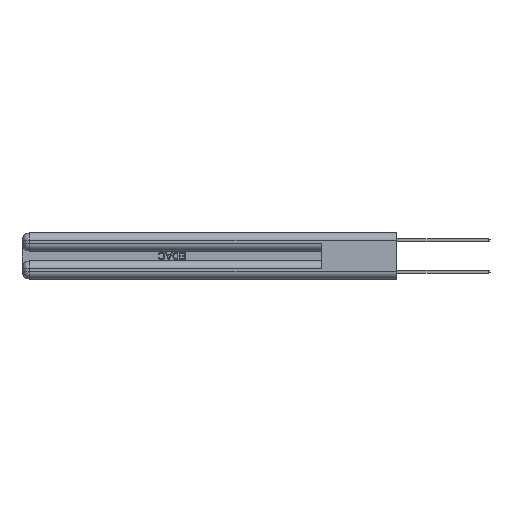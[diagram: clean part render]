
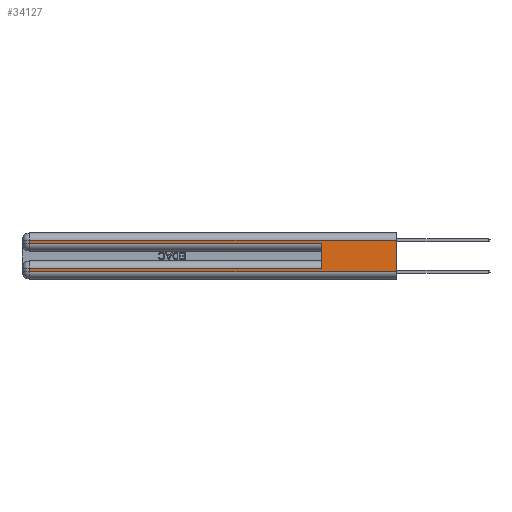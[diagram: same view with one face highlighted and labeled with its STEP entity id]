
A CAD part, left-side view. The second image highlights one B-rep face of the part: STEP entity #34127.
In plain terms, the highlighted planar face has unit normal (-1, 0, 0).
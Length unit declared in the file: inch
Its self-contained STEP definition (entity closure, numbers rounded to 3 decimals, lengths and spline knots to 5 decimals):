
#540 = EDGE_CURVE ( 'NONE', #30576, #14125, #21364, .T. ) ;
#1608 = ORIENTED_EDGE ( 'NONE', *, *, #540, .F. ) ;
#1637 = DIRECTION ( 'NONE',  ( 0., 1., 0. ) ) ;
#1797 = DIRECTION ( 'NONE',  ( 1., 0., 0. ) ) ;
#2330 = CARTESIAN_POINT ( 'NONE',  ( 0., 2.94, 0.31 ) ) ;
#2405 = CARTESIAN_POINT ( 'NONE',  ( 0., 2.94, 0.085 ) ) ;
#2927 = EDGE_LOOP ( 'NONE', ( #27603, #15853, #14263, #14037, #1608, #10735, #12946, #26251 ) ) ;
#3927 = PLANE ( 'NONE',  #29278 ) ;
#5825 = EDGE_CURVE ( 'NONE', #24132, #31583, #33546, .T. ) ;
#5910 = DIRECTION ( 'NONE',  ( 0., 0., -1. ) ) ;
#6086 = CARTESIAN_POINT ( 'NONE',  ( 0., 0., 0.085 ) ) ;
#7013 = DIRECTION ( 'NONE',  ( 0., 0., -1. ) ) ;
#7565 = VECTOR ( 'NONE', #11944, 39.37008 ) ;
#7853 = VECTOR ( 'NONE', #16597, 39.37008 ) ;
#8237 = EDGE_CURVE ( 'NONE', #31583, #25192, #31632, .T. ) ;
#10208 = CARTESIAN_POINT ( 'NONE',  ( 0., 0., 0.31 ) ) ;
#10735 = ORIENTED_EDGE ( 'NONE', *, *, #13315, .T. ) ;
#11313 = VERTEX_POINT ( 'NONE', #2330 ) ;
#11636 = CARTESIAN_POINT ( 'NONE',  ( 0., 0., 0.37 ) ) ;
#11944 = DIRECTION ( 'NONE',  ( 0., 0., -1. ) ) ;
#12946 = ORIENTED_EDGE ( 'NONE', *, *, #5825, .T. ) ;
#13315 = EDGE_CURVE ( 'NONE', #30576, #24132, #30402, .T. ) ;
#13372 = EDGE_CURVE ( 'NONE', #11313, #16018, #21155, .T. ) ;
#13816 = FACE_OUTER_BOUND ( 'NONE', #2927, .T. ) ;
#13921 = DIRECTION ( 'NONE',  ( 0., -1., 0. ) ) ;
#14037 = ORIENTED_EDGE ( 'NONE', *, *, #24887, .T. ) ;
#14125 = VERTEX_POINT ( 'NONE', #23801 ) ;
#14263 = ORIENTED_EDGE ( 'NONE', *, *, #13372, .T. ) ;
#14630 = CARTESIAN_POINT ( 'NONE',  ( 0., 0., 0.285 ) ) ;
#15293 = EDGE_CURVE ( 'NONE', #24166, #11313, #15877, .T. ) ;
#15853 = ORIENTED_EDGE ( 'NONE', *, *, #15293, .T. ) ;
#15877 = LINE ( 'NONE', #10208, #29428 ) ;
#16018 = VERTEX_POINT ( 'NONE', #25874 ) ;
#16597 = DIRECTION ( 'NONE',  ( 0., 0., -1. ) ) ;
#16702 = CARTESIAN_POINT ( 'NONE',  ( 0., 2.94, 0.37 ) ) ;
#16975 = CARTESIAN_POINT ( 'NONE',  ( 0., 2.94, 0.06 ) ) ;
#20719 = VECTOR ( 'NONE', #30306, 39.37008 ) ;
#21155 = LINE ( 'NONE', #16702, #7853 ) ;
#21364 = LINE ( 'NONE', #31887, #34923 ) ;
#22995 = CARTESIAN_POINT ( 'NONE',  ( 0., 0., 0.37 ) ) ;
#23801 = CARTESIAN_POINT ( 'NONE',  ( 0., 0.6, 0.285 ) ) ;
#23851 = DIRECTION ( 'NONE',  ( 0., 0., 1. ) ) ;
#24132 = VERTEX_POINT ( 'NONE', #2405 ) ;
#24166 = VERTEX_POINT ( 'NONE', #29733 ) ;
#24633 = CARTESIAN_POINT ( 'NONE',  ( 0., 0., 0.06 ) ) ;
#24721 = CARTESIAN_POINT ( 'NONE',  ( 0., 0.6, 0.085 ) ) ;
#24887 = EDGE_CURVE ( 'NONE', #16018, #14125, #33548, .T. ) ;
#25192 = VERTEX_POINT ( 'NONE', #27839 ) ;
#25874 = CARTESIAN_POINT ( 'NONE',  ( 0., 2.94, 0.285 ) ) ;
#26251 = ORIENTED_EDGE ( 'NONE', *, *, #8237, .T. ) ;
#27603 = ORIENTED_EDGE ( 'NONE', *, *, #27708, .F. ) ;
#27708 = EDGE_CURVE ( 'NONE', #24166, #25192, #32959, .T. ) ;
#27839 = CARTESIAN_POINT ( 'NONE',  ( 0., 0., 0.06 ) ) ;
#29278 = AXIS2_PLACEMENT_3D ( 'NONE', #22995, #1797, #7013 ) ;
#29428 = VECTOR ( 'NONE', #1637, 39.37008 ) ;
#29511 = VECTOR ( 'NONE', #13921, 39.37008 ) ;
#29733 = CARTESIAN_POINT ( 'NONE',  ( 0., 0., 0.31 ) ) ;
#30306 = DIRECTION ( 'NONE',  ( 0., 1., 0. ) ) ;
#30402 = LINE ( 'NONE', #6086, #20719 ) ;
#30576 = VERTEX_POINT ( 'NONE', #24721 ) ;
#30774 = CARTESIAN_POINT ( 'NONE',  ( 0., 2.94, 0.37 ) ) ;
#31583 = VERTEX_POINT ( 'NONE', #16975 ) ;
#31632 = LINE ( 'NONE', #24633, #29511 ) ;
#31848 = VECTOR ( 'NONE', #33750, 39.37008 ) ;
#31887 = CARTESIAN_POINT ( 'NONE',  ( 0., 0.6, 0.145 ) ) ;
#32959 = LINE ( 'NONE', #11636, #35102 ) ;
#33546 = LINE ( 'NONE', #30774, #7565 ) ;
#33548 = LINE ( 'NONE', #14630, #31848 ) ;
#33750 = DIRECTION ( 'NONE',  ( 0., -1., 0. ) ) ;
#34127 = ADVANCED_FACE ( 'NONE', ( #13816 ), #3927, .F. ) ;
#34923 = VECTOR ( 'NONE', #23851, 39.37008 ) ;
#35102 = VECTOR ( 'NONE', #5910, 39.37008 ) ;
